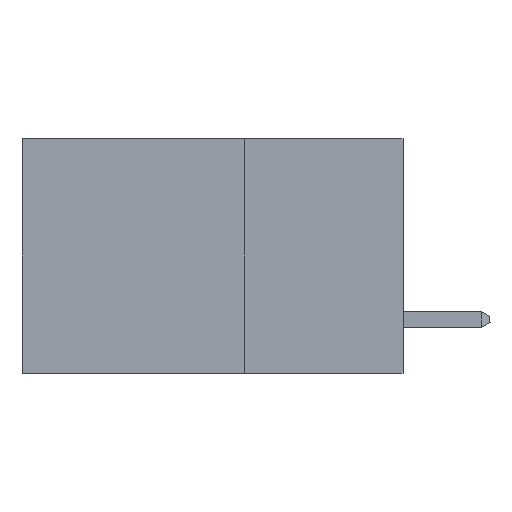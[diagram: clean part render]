
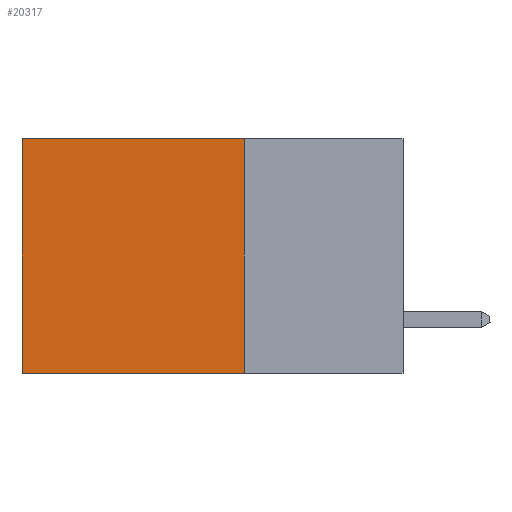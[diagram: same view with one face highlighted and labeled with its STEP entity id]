
A CAD part, left-side view. The second image highlights one B-rep face of the part: STEP entity #20317.
In plain terms, the highlighted planar face has unit normal (-1, 0, 0).
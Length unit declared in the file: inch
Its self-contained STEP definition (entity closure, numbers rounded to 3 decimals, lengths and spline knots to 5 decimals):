
#377 = VECTOR ( 'NONE', #20133, 39.37008 ) ;
#2079 = DIRECTION ( 'NONE',  ( 0., 1., 0. ) ) ;
#2283 = EDGE_CURVE ( 'NONE', #15196, #24113, #11858, .T. ) ;
#2345 = CARTESIAN_POINT ( 'NONE',  ( 0.2875, 0.25, 0. ) ) ;
#2516 = PLANE ( 'NONE',  #16774 ) ;
#2929 = DIRECTION ( 'NONE',  ( 0., 0., -1. ) ) ;
#3196 = LINE ( 'NONE', #29607, #30347 ) ;
#3858 = DIRECTION ( 'NONE',  ( 0., 0., -1. ) ) ;
#3994 = CARTESIAN_POINT ( 'NONE',  ( 0.2875, 0.25, 0. ) ) ;
#5673 = ORIENTED_EDGE ( 'NONE', *, *, #20633, .T. ) ;
#5884 = CARTESIAN_POINT ( 'NONE',  ( 0.2875, 0.6, 0. ) ) ;
#8013 = CARTESIAN_POINT ( 'NONE',  ( 0.2875, 0.6, -0.37 ) ) ;
#9573 = CARTESIAN_POINT ( 'NONE',  ( 0.2875, 0.25, 0. ) ) ;
#9681 = DIRECTION ( 'NONE',  ( 1., 0., 0. ) ) ;
#9833 = VERTEX_POINT ( 'NONE', #29677 ) ;
#11047 = EDGE_CURVE ( 'NONE', #18209, #15196, #3196, .T. ) ;
#11809 = EDGE_LOOP ( 'NONE', ( #5673, #22307, #27170, #12716 ) ) ;
#11858 = LINE ( 'NONE', #14087, #23241 ) ;
#12716 = ORIENTED_EDGE ( 'NONE', *, *, #14061, .T. ) ;
#14061 = EDGE_CURVE ( 'NONE', #18209, #9833, #26064, .T. ) ;
#14087 = CARTESIAN_POINT ( 'NONE',  ( 0.2875, 0.25, -0.37 ) ) ;
#14845 = CARTESIAN_POINT ( 'NONE',  ( 0.2875, 0.25, -0.37 ) ) ;
#15196 = VERTEX_POINT ( 'NONE', #14845 ) ;
#16774 = AXIS2_PLACEMENT_3D ( 'NONE', #9573, #9681, #2929 ) ;
#18209 = VERTEX_POINT ( 'NONE', #3994 ) ;
#20133 = DIRECTION ( 'NONE',  ( 0., 1., 0. ) ) ;
#20317 = ADVANCED_FACE ( 'NONE', ( #21778 ), #2516, .F. ) ;
#20633 = EDGE_CURVE ( 'NONE', #9833, #24113, #24449, .T. ) ;
#21778 = FACE_OUTER_BOUND ( 'NONE', #11809, .T. ) ;
#22307 = ORIENTED_EDGE ( 'NONE', *, *, #2283, .F. ) ;
#23241 = VECTOR ( 'NONE', #2079, 39.37008 ) ;
#24113 = VERTEX_POINT ( 'NONE', #8013 ) ;
#24449 = LINE ( 'NONE', #5884, #28534 ) ;
#24762 = DIRECTION ( 'NONE',  ( 0., 0., -1. ) ) ;
#26064 = LINE ( 'NONE', #2345, #377 ) ;
#27170 = ORIENTED_EDGE ( 'NONE', *, *, #11047, .F. ) ;
#28534 = VECTOR ( 'NONE', #24762, 39.37008 ) ;
#29607 = CARTESIAN_POINT ( 'NONE',  ( 0.2875, 0.25, 0. ) ) ;
#29677 = CARTESIAN_POINT ( 'NONE',  ( 0.2875, 0.6, 0. ) ) ;
#30347 = VECTOR ( 'NONE', #3858, 39.37008 ) ;
